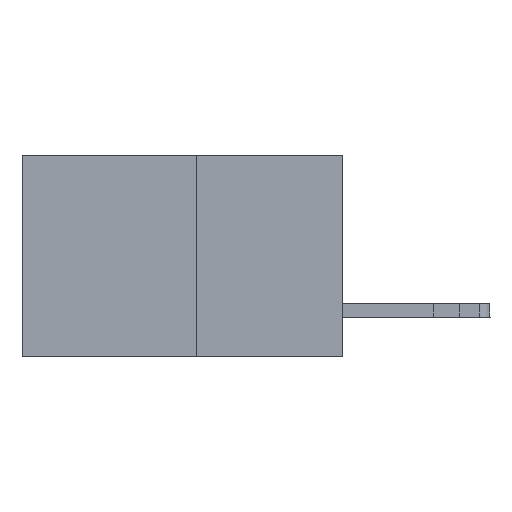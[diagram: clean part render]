
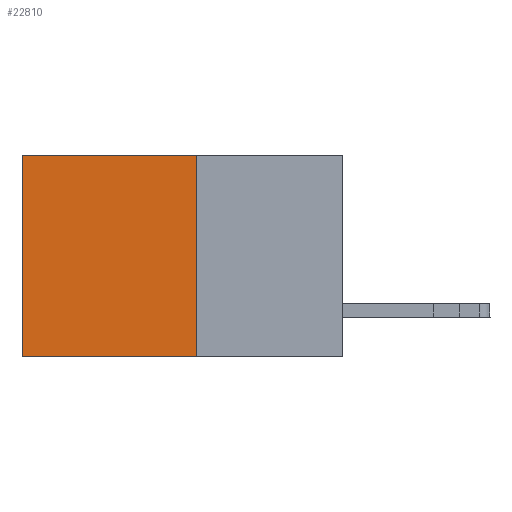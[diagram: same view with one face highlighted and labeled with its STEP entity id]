
A CAD part, left-side view. The second image highlights one B-rep face of the part: STEP entity #22810.
In plain terms, the highlighted planar face has unit normal (-1, 0, 0).
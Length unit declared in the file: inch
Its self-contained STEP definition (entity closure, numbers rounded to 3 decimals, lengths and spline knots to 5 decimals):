
#481 = LINE ( 'NONE', #15448, #15484 ) ;
#1366 = CARTESIAN_POINT ( 'NONE',  ( 0.277, 0.59, 0. ) ) ;
#1831 = DIRECTION ( 'NONE',  ( 0., 1., 0. ) ) ;
#2449 = DIRECTION ( 'NONE',  ( 0., 0., -1. ) ) ;
#3445 = VERTEX_POINT ( 'NONE', #19045 ) ;
#3491 = PLANE ( 'NONE',  #7596 ) ;
#3647 = CARTESIAN_POINT ( 'NONE',  ( 0.277, 0.27, 0. ) ) ;
#6074 = CARTESIAN_POINT ( 'NONE',  ( 0.277, 0.27, -0.37 ) ) ;
#6149 = DIRECTION ( 'NONE',  ( 0., 0., -1. ) ) ;
#7222 = VECTOR ( 'NONE', #2449, 39.37008 ) ;
#7596 = AXIS2_PLACEMENT_3D ( 'NONE', #16365, #23878, #10959 ) ;
#9313 = ORIENTED_EDGE ( 'NONE', *, *, #16273, .F. ) ;
#9985 = EDGE_CURVE ( 'NONE', #18157, #3445, #481, .T. ) ;
#10008 = VERTEX_POINT ( 'NONE', #23982 ) ;
#10306 = ORIENTED_EDGE ( 'NONE', *, *, #9985, .T. ) ;
#10959 = DIRECTION ( 'NONE',  ( 0., 0., -1. ) ) ;
#10995 = EDGE_LOOP ( 'NONE', ( #10306, #9313, #19234, #12497 ) ) ;
#11021 = VERTEX_POINT ( 'NONE', #17714 ) ;
#11071 = FACE_OUTER_BOUND ( 'NONE', #10995, .T. ) ;
#12497 = ORIENTED_EDGE ( 'NONE', *, *, #17587, .T. ) ;
#13541 = DIRECTION ( 'NONE',  ( 0., 1., 0. ) ) ;
#14314 = VECTOR ( 'NONE', #13541, 39.37008 ) ;
#15448 = CARTESIAN_POINT ( 'NONE',  ( 0.277, 0.59, -0.37 ) ) ;
#15484 = VECTOR ( 'NONE', #6149, 39.37008 ) ;
#16273 = EDGE_CURVE ( 'NONE', #11021, #3445, #22892, .T. ) ;
#16365 = CARTESIAN_POINT ( 'NONE',  ( 0.277, 0.27, -0.37 ) ) ;
#17587 = EDGE_CURVE ( 'NONE', #10008, #18157, #20453, .T. ) ;
#17714 = CARTESIAN_POINT ( 'NONE',  ( 0.277, 0.27, -0.37 ) ) ;
#18157 = VERTEX_POINT ( 'NONE', #1366 ) ;
#19045 = CARTESIAN_POINT ( 'NONE',  ( 0.277, 0.59, -0.37 ) ) ;
#19234 = ORIENTED_EDGE ( 'NONE', *, *, #22086, .F. ) ;
#19246 = LINE ( 'NONE', #22514, #7222 ) ;
#20453 = LINE ( 'NONE', #3647, #20613 ) ;
#20613 = VECTOR ( 'NONE', #1831, 39.37008 ) ;
#22086 = EDGE_CURVE ( 'NONE', #10008, #11021, #19246, .T. ) ;
#22514 = CARTESIAN_POINT ( 'NONE',  ( 0.277, 0.27, -0.37 ) ) ;
#22810 = ADVANCED_FACE ( 'NONE', ( #11071 ), #3491, .F. ) ;
#22892 = LINE ( 'NONE', #6074, #14314 ) ;
#23878 = DIRECTION ( 'NONE',  ( 1., 0., 0. ) ) ;
#23982 = CARTESIAN_POINT ( 'NONE',  ( 0.277, 0.27, 0. ) ) ;
